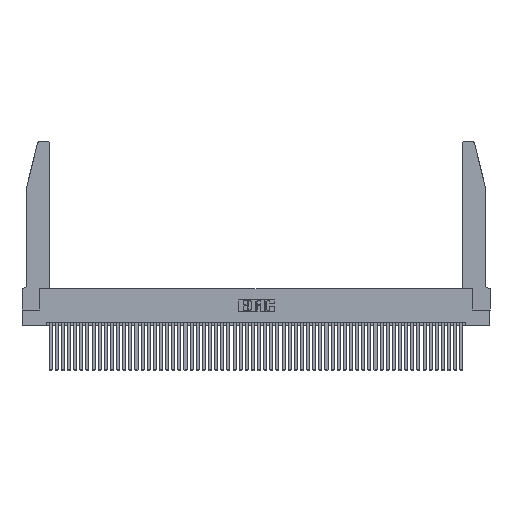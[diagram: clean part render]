
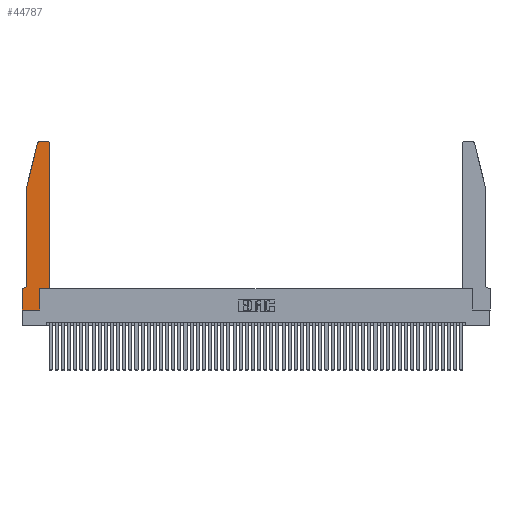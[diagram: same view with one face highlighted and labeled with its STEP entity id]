
A CAD part, top view. The second image highlights one B-rep face of the part: STEP entity #44787.
In plain terms, the highlighted planar face has unit normal (0, 0, 1).
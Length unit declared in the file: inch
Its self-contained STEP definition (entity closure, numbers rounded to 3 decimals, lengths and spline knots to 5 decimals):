
#319 = CARTESIAN_POINT ( 'NONE',  ( 0.0055, 0.42, 0.37 ) ) ;
#1344 = ORIENTED_EDGE ( 'NONE', *, *, #25343, .T. ) ;
#2667 = CARTESIAN_POINT ( 'NONE',  ( 0.4205, 2.72, 0.37 ) ) ;
#2875 = EDGE_CURVE ( 'NONE', #14598, #23839, #16706, .T. ) ;
#3574 = CARTESIAN_POINT ( 'NONE',  ( 0.4505, 0.35, 0.37 ) ) ;
#4594 = DIRECTION ( 'NONE',  ( -1., 0., 0. ) ) ;
#4922 = LINE ( 'NONE', #29882, #46559 ) ;
#4924 = ORIENTED_EDGE ( 'NONE', *, *, #27495, .T. ) ;
#6929 = DIRECTION ( 'NONE',  ( 1., 0., 0. ) ) ;
#6992 = LINE ( 'NONE', #16580, #18355 ) ;
#7852 = DIRECTION ( 'NONE',  ( 0., 1., 0. ) ) ;
#8939 = DIRECTION ( 'NONE',  ( 0., -1., 0. ) ) ;
#9076 = VERTEX_POINT ( 'NONE', #52999 ) ;
#9670 = CARTESIAN_POINT ( 'NONE',  ( 0.4205, 2.75, 0.37 ) ) ;
#9687 = VERTEX_POINT ( 'NONE', #23408 ) ;
#10372 = CARTESIAN_POINT ( 'NONE',  ( 0., 0., 0.37 ) ) ;
#10374 = CARTESIAN_POINT ( 'NONE',  ( 0.4505, 0.35, 0.37 ) ) ;
#10431 = CARTESIAN_POINT ( 'NONE',  ( 0.0055, 0.35, 0.37 ) ) ;
#12265 = LINE ( 'NONE', #37887, #52918 ) ;
#12569 = CARTESIAN_POINT ( 'NONE',  ( 0.25487, 2.72718, 0.37 ) ) ;
#12771 = CIRCLE ( 'NONE', #52957, 0.03 ) ;
#13179 = DIRECTION ( 'NONE',  ( -1., 0., 0. ) ) ;
#13736 = EDGE_CURVE ( 'NONE', #9076, #52848, #52647, .T. ) ;
#13884 = VERTEX_POINT ( 'NONE', #15585 ) ;
#14598 = VERTEX_POINT ( 'NONE', #34448 ) ;
#14610 = LINE ( 'NONE', #3574, #44209 ) ;
#14658 = DIRECTION ( 'NONE',  ( 1., 0., 0. ) ) ;
#14667 = VERTEX_POINT ( 'NONE', #9670 ) ;
#14676 = CARTESIAN_POINT ( 'NONE',  ( 0.0755, 0.42, 0.37 ) ) ;
#15585 = CARTESIAN_POINT ( 'NONE',  ( 0.0755, 2., 0.37 ) ) ;
#16580 = CARTESIAN_POINT ( 'NONE',  ( 0.0755, 2., 0.37 ) ) ;
#16706 = CIRCLE ( 'NONE', #16964, 0.03 ) ;
#16964 = AXIS2_PLACEMENT_3D ( 'NONE', #45532, #20442, #49678 ) ;
#18100 = CARTESIAN_POINT ( 'NONE',  ( 0.2865, 0., 0.37 ) ) ;
#18283 = CIRCLE ( 'NONE', #43166, 0.07 ) ;
#18355 = VECTOR ( 'NONE', #41587, 39.37008 ) ;
#18486 = ORIENTED_EDGE ( 'NONE', *, *, #26149, .T. ) ;
#18689 = CARTESIAN_POINT ( 'NONE',  ( 0.2865, 0.35, 0.37 ) ) ;
#18970 = VERTEX_POINT ( 'NONE', #31219 ) ;
#19268 = DIRECTION ( 'NONE',  ( 0., 0., 1. ) ) ;
#19343 = VECTOR ( 'NONE', #35839, 39.37008 ) ;
#19958 = ORIENTED_EDGE ( 'NONE', *, *, #44996, .T. ) ;
#20442 = DIRECTION ( 'NONE',  ( 0., 0., 1. ) ) ;
#20547 = ORIENTED_EDGE ( 'NONE', *, *, #33494, .T. ) ;
#21155 = LINE ( 'NONE', #31645, #42159 ) ;
#21178 = DIRECTION ( 'NONE',  ( 0., 1., 0. ) ) ;
#21947 = ORIENTED_EDGE ( 'NONE', *, *, #50832, .T. ) ;
#23408 = CARTESIAN_POINT ( 'NONE',  ( 0., 0.35, 0.37 ) ) ;
#23839 = VERTEX_POINT ( 'NONE', #12569 ) ;
#25062 = VECTOR ( 'NONE', #14658, 39.37008 ) ;
#25164 = CARTESIAN_POINT ( 'NONE',  ( 0.4505, 0.35, 0.37 ) ) ;
#25343 = EDGE_CURVE ( 'NONE', #52996, #9687, #21155, .T. ) ;
#25553 = DIRECTION ( 'NONE',  ( 0., -1., 0. ) ) ;
#25777 = CARTESIAN_POINT ( 'NONE',  ( 0.2605, 2.75, 0.37 ) ) ;
#25938 = ORIENTED_EDGE ( 'NONE', *, *, #13736, .T. ) ;
#26149 = EDGE_CURVE ( 'NONE', #9687, #9076, #48539, .T. ) ;
#27495 = EDGE_CURVE ( 'NONE', #23839, #13884, #6992, .T. ) ;
#27532 = CARTESIAN_POINT ( 'NONE',  ( 0., 0.35, 0.37 ) ) ;
#29882 = CARTESIAN_POINT ( 'NONE',  ( 0.0755, 2., 0.37 ) ) ;
#29985 = DIRECTION ( 'NONE',  ( 0., 0., -1. ) ) ;
#31219 = CARTESIAN_POINT ( 'NONE',  ( 0.4505, 2.72, 0.37 ) ) ;
#31645 = CARTESIAN_POINT ( 'NONE',  ( 0.0755, 0.35, 0.37 ) ) ;
#31847 = VERTEX_POINT ( 'NONE', #18689 ) ;
#32322 = DIRECTION ( 'NONE',  ( 0., 0., 1. ) ) ;
#33494 = EDGE_CURVE ( 'NONE', #14667, #14598, #49735, .T. ) ;
#33788 = FACE_OUTER_BOUND ( 'NONE', #37334, .T. ) ;
#34448 = CARTESIAN_POINT ( 'NONE',  ( 0.284, 2.75, 0.37 ) ) ;
#34851 = VECTOR ( 'NONE', #25553, 39.37008 ) ;
#35319 = ORIENTED_EDGE ( 'NONE', *, *, #38437, .T. ) ;
#35664 = DIRECTION ( 'NONE',  ( -1., 0., 0. ) ) ;
#35839 = DIRECTION ( 'NONE',  ( 1., 0., 0. ) ) ;
#37334 = EDGE_LOOP ( 'NONE', ( #20547, #40789, #4924, #21947, #35319, #1344, #18486, #25938, #48415, #45671, #19958, #49528 ) ) ;
#37887 = CARTESIAN_POINT ( 'NONE',  ( 0.2865, 0.35, 0.37 ) ) ;
#38361 = EDGE_CURVE ( 'NONE', #52848, #31847, #12265, .T. ) ;
#38437 = EDGE_CURVE ( 'NONE', #40039, #52996, #18283, .T. ) ;
#38442 = AXIS2_PLACEMENT_3D ( 'NONE', #27532, #19268, #48530 ) ;
#38700 = VECTOR ( 'NONE', #13179, 39.37008 ) ;
#38857 = LINE ( 'NONE', #10374, #25062 ) ;
#40039 = VERTEX_POINT ( 'NONE', #14676 ) ;
#40789 = ORIENTED_EDGE ( 'NONE', *, *, #2875, .T. ) ;
#41587 = DIRECTION ( 'NONE',  ( -0.239, -0.971, 0. ) ) ;
#42159 = VECTOR ( 'NONE', #35664, 39.37008 ) ;
#42747 = EDGE_CURVE ( 'NONE', #18970, #14667, #12771, .T. ) ;
#43166 = AXIS2_PLACEMENT_3D ( 'NONE', #319, #29985, #4594 ) ;
#44209 = VECTOR ( 'NONE', #7852, 39.37008 ) ;
#44378 = PLANE ( 'NONE',  #38442 ) ;
#44787 = ADVANCED_FACE ( 'NONE', ( #33788 ), #44378, .T. ) ;
#44996 = EDGE_CURVE ( 'NONE', #46268, #18970, #14610, .T. ) ;
#45532 = CARTESIAN_POINT ( 'NONE',  ( 0.284, 2.72, 0.37 ) ) ;
#45671 = ORIENTED_EDGE ( 'NONE', *, *, #49022, .T. ) ;
#46268 = VERTEX_POINT ( 'NONE', #25164 ) ;
#46413 = CARTESIAN_POINT ( 'NONE',  ( 0., 0., 0.37 ) ) ;
#46559 = VECTOR ( 'NONE', #8939, 39.37008 ) ;
#48415 = ORIENTED_EDGE ( 'NONE', *, *, #38361, .T. ) ;
#48530 = DIRECTION ( 'NONE',  ( 1., 0., 0. ) ) ;
#48539 = LINE ( 'NONE', #46413, #34851 ) ;
#49022 = EDGE_CURVE ( 'NONE', #31847, #46268, #38857, .T. ) ;
#49528 = ORIENTED_EDGE ( 'NONE', *, *, #42747, .T. ) ;
#49678 = DIRECTION ( 'NONE',  ( 1., 0., 0. ) ) ;
#49735 = LINE ( 'NONE', #25777, #38700 ) ;
#50832 = EDGE_CURVE ( 'NONE', #13884, #40039, #4922, .T. ) ;
#52647 = LINE ( 'NONE', #10372, #19343 ) ;
#52848 = VERTEX_POINT ( 'NONE', #18100 ) ;
#52918 = VECTOR ( 'NONE', #21178, 39.37008 ) ;
#52957 = AXIS2_PLACEMENT_3D ( 'NONE', #2667, #32322, #6929 ) ;
#52996 = VERTEX_POINT ( 'NONE', #10431 ) ;
#52999 = CARTESIAN_POINT ( 'NONE',  ( 0., 0., 0.37 ) ) ;
